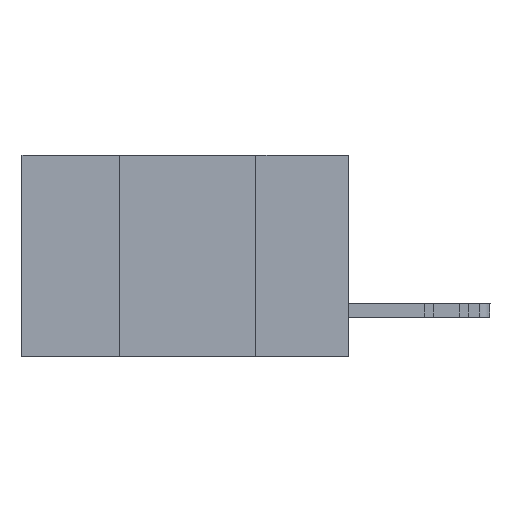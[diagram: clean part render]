
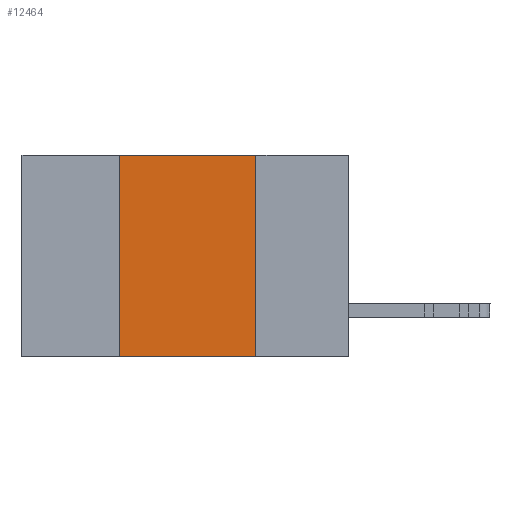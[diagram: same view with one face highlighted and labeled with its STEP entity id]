
A CAD part, left-side view. The second image highlights one B-rep face of the part: STEP entity #12464.
In plain terms, the highlighted planar face has unit normal (-1, 0, 0).
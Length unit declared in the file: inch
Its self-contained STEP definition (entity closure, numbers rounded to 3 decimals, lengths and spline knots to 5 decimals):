
#1218 = CARTESIAN_POINT ( 'NONE',  ( 0., 0.6, 0. ) ) ;
#1971 = VECTOR ( 'NONE', #10507, 39.37008 ) ;
#2487 = VERTEX_POINT ( 'NONE', #27640 ) ;
#2538 = FACE_OUTER_BOUND ( 'NONE', #19889, .T. ) ;
#2721 = DIRECTION ( 'NONE',  ( 1., 0., 0. ) ) ;
#2956 = VERTEX_POINT ( 'NONE', #12798 ) ;
#2983 = AXIS2_PLACEMENT_3D ( 'NONE', #25165, #2721, #30439 ) ;
#3589 = DIRECTION ( 'NONE',  ( 0., -1., 0. ) ) ;
#3937 = ORIENTED_EDGE ( 'NONE', *, *, #23121, .F. ) ;
#4315 = VECTOR ( 'NONE', #8795, 39.37008 ) ;
#5097 = VECTOR ( 'NONE', #6570, 39.37008 ) ;
#6439 = VERTEX_POINT ( 'NONE', #16004 ) ;
#6570 = DIRECTION ( 'NONE',  ( 0., 0., 1. ) ) ;
#6654 = CARTESIAN_POINT ( 'NONE',  ( 0., 0.17, 0. ) ) ;
#6678 = VERTEX_POINT ( 'NONE', #16181 ) ;
#7872 = EDGE_CURVE ( 'NONE', #6439, #2956, #27794, .T. ) ;
#8310 = EDGE_CURVE ( 'NONE', #6678, #6439, #31655, .T. ) ;
#8795 = DIRECTION ( 'NONE',  ( 0., 0., -1. ) ) ;
#10021 = EDGE_CURVE ( 'NONE', #6678, #2487, #27316, .T. ) ;
#10507 = DIRECTION ( 'NONE',  ( 0., -1., 0. ) ) ;
#10758 = ORIENTED_EDGE ( 'NONE', *, *, #8310, .F. ) ;
#12464 = ADVANCED_FACE ( 'NONE', ( #2538 ), #17550, .F. ) ;
#12798 = CARTESIAN_POINT ( 'NONE',  ( 0., 0.17, 0. ) ) ;
#14071 = CARTESIAN_POINT ( 'NONE',  ( 0., 0.42, 0. ) ) ;
#16004 = CARTESIAN_POINT ( 'NONE',  ( 0., 0.42, 0. ) ) ;
#16181 = CARTESIAN_POINT ( 'NONE',  ( 0., 0.42, -0.37 ) ) ;
#17550 = PLANE ( 'NONE',  #2983 ) ;
#18028 = CARTESIAN_POINT ( 'NONE',  ( 0., 0.6, -0.37 ) ) ;
#19568 = ORIENTED_EDGE ( 'NONE', *, *, #10021, .T. ) ;
#19889 = EDGE_LOOP ( 'NONE', ( #3937, #20385, #10758, #19568 ) ) ;
#20385 = ORIENTED_EDGE ( 'NONE', *, *, #7872, .F. ) ;
#23121 = EDGE_CURVE ( 'NONE', #2956, #2487, #28548, .T. ) ;
#25165 = CARTESIAN_POINT ( 'NONE',  ( 0., 0.6, 0. ) ) ;
#26689 = VECTOR ( 'NONE', #3589, 39.37008 ) ;
#27316 = LINE ( 'NONE', #18028, #1971 ) ;
#27640 = CARTESIAN_POINT ( 'NONE',  ( 0., 0.17, -0.37 ) ) ;
#27794 = LINE ( 'NONE', #1218, #26689 ) ;
#28548 = LINE ( 'NONE', #6654, #4315 ) ;
#30439 = DIRECTION ( 'NONE',  ( 0., 0., -1. ) ) ;
#31655 = LINE ( 'NONE', #14071, #5097 ) ;
